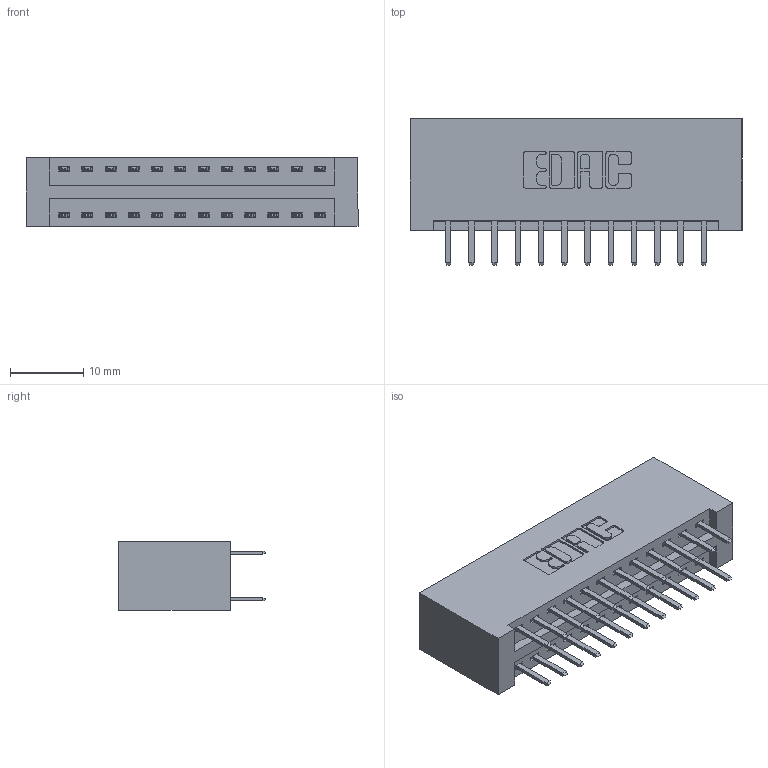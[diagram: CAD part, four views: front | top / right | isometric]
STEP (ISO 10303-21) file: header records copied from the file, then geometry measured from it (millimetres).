
FILE_DESCRIPTION (( 'STEP AP203' ), '1' );
FILE_NAME ('396-024-520-201.STEP', '2018-09-01T12:34:06', ( '' ), ( '' ), 'SwSTEP 2.0', 'SolidWorks 2016', '' );
FILE_SCHEMA (( 'CONFIG_CONTROL_DESIGN' ));
Length unit declared in the file: inch
Products named in the file (3): 346 Part_No Mounting Lugs; 345-292-001_345-293-120; 396-024-520-201
Assembly tree (25 placements, depth 2):
  396-024-520-201
    346 Part_No Mounting Lugs
    345-292-001_345-293-120  x24
Bounding box: 45.34 x 20.02 x 9.4 mm (x, y, z)
Volume: 4750.8 mm3; surface area: 6197.3 mm2
Topology: 25 solids, 25 shells, 1458 faces, 4217 edges, 2746 vertices
Faces by surface type: plane 960, cylinder 498
Entity records: 11707 total; most frequent: CARTESIAN_POINT 1980, ORIENTED_EDGE 1902, DIRECTION 1779, EDGE_CURVE 951, VECTOR 775, LINE 775, VERTEX_POINT 630, AXIS2_PLACEMENT_3D 502
